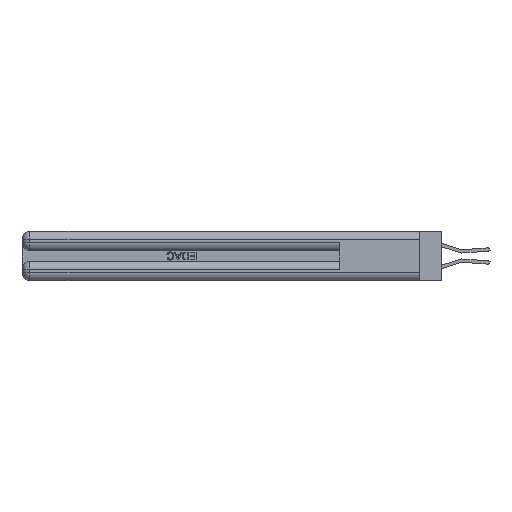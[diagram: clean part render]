
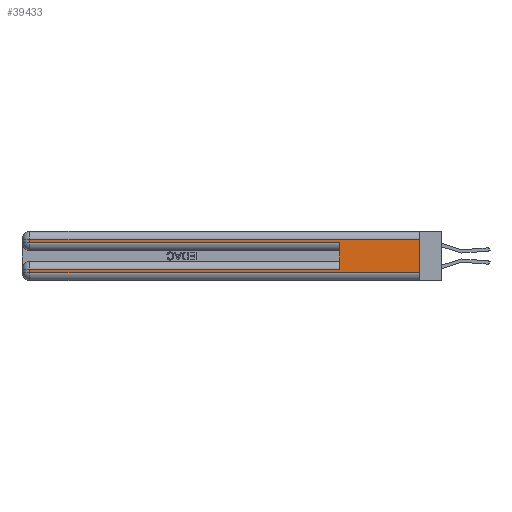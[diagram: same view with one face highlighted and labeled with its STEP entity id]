
A CAD part, left-side view. The second image highlights one B-rep face of the part: STEP entity #39433.
In plain terms, the highlighted planar face has unit normal (-1, 0, 0).
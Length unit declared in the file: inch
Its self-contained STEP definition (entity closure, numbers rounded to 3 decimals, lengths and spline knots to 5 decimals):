
#212 = EDGE_LOOP ( 'NONE', ( #5821, #11777, #9363, #39288, #15627, #4521, #4432, #2448 ) ) ;
#585 = EDGE_CURVE ( 'NONE', #40706, #16194, #4426, .T. ) ;
#684 = VECTOR ( 'NONE', #37307, 39.37008 ) ;
#828 = CARTESIAN_POINT ( 'NONE',  ( 0., 0., 0.06 ) ) ;
#2060 = VERTEX_POINT ( 'NONE', #25319 ) ;
#2448 = ORIENTED_EDGE ( 'NONE', *, *, #4503, .T. ) ;
#3574 = LINE ( 'NONE', #6690, #38582 ) ;
#3845 = CARTESIAN_POINT ( 'NONE',  ( 0., 0.6, 0.145 ) ) ;
#4426 = LINE ( 'NONE', #31833, #6719 ) ;
#4432 = ORIENTED_EDGE ( 'NONE', *, *, #28963, .T. ) ;
#4503 = EDGE_CURVE ( 'NONE', #17765, #16194, #44807, .T. ) ;
#4521 = ORIENTED_EDGE ( 'NONE', *, *, #9127, .T. ) ;
#4641 = LINE ( 'NONE', #33483, #684 ) ;
#4909 = DIRECTION ( 'NONE',  ( 0., -1., 0. ) ) ;
#5194 = CARTESIAN_POINT ( 'NONE',  ( 0., 0.6, 0.085 ) ) ;
#5243 = VERTEX_POINT ( 'NONE', #29019 ) ;
#5821 = ORIENTED_EDGE ( 'NONE', *, *, #585, .F. ) ;
#6690 = CARTESIAN_POINT ( 'NONE',  ( 0., 2.94, 0.37 ) ) ;
#6719 = VECTOR ( 'NONE', #18089, 39.37008 ) ;
#7585 = VECTOR ( 'NONE', #30262, 39.37008 ) ;
#8351 = VERTEX_POINT ( 'NONE', #16807 ) ;
#8817 = CARTESIAN_POINT ( 'NONE',  ( 0., 0., 0.285 ) ) ;
#9003 = VECTOR ( 'NONE', #21394, 39.37008 ) ;
#9127 = EDGE_CURVE ( 'NONE', #21101, #5243, #4641, .T. ) ;
#9363 = ORIENTED_EDGE ( 'NONE', *, *, #11180, .T. ) ;
#11180 = EDGE_CURVE ( 'NONE', #25715, #2060, #43807, .T. ) ;
#11777 = ORIENTED_EDGE ( 'NONE', *, *, #38386, .T. ) ;
#13094 = VECTOR ( 'NONE', #4909, 39.37008 ) ;
#15627 = ORIENTED_EDGE ( 'NONE', *, *, #40161, .F. ) ;
#15644 = VECTOR ( 'NONE', #36802, 39.37008 ) ;
#15941 = VECTOR ( 'NONE', #24783, 39.37008 ) ;
#16194 = VERTEX_POINT ( 'NONE', #828 ) ;
#16807 = CARTESIAN_POINT ( 'NONE',  ( 0., 0.6, 0.285 ) ) ;
#17201 = CARTESIAN_POINT ( 'NONE',  ( 0., 0., 0.06 ) ) ;
#17765 = VERTEX_POINT ( 'NONE', #37957 ) ;
#18089 = DIRECTION ( 'NONE',  ( 0., 0., -1. ) ) ;
#18443 = LINE ( 'NONE', #3845, #15644 ) ;
#21101 = VERTEX_POINT ( 'NONE', #5194 ) ;
#21394 = DIRECTION ( 'NONE',  ( 0., 1., 0. ) ) ;
#22194 = CARTESIAN_POINT ( 'NONE',  ( 0., 2.94, 0.37 ) ) ;
#24700 = DIRECTION ( 'NONE',  ( 0., 0., -1. ) ) ;
#24783 = DIRECTION ( 'NONE',  ( 0., -1., 0. ) ) ;
#24889 = CARTESIAN_POINT ( 'NONE',  ( 0., 0., 0.31 ) ) ;
#25319 = CARTESIAN_POINT ( 'NONE',  ( 0., 2.94, 0.285 ) ) ;
#25715 = VERTEX_POINT ( 'NONE', #43139 ) ;
#28435 = CARTESIAN_POINT ( 'NONE',  ( 0., 0., 0.31 ) ) ;
#28963 = EDGE_CURVE ( 'NONE', #5243, #17765, #3574, .T. ) ;
#29019 = CARTESIAN_POINT ( 'NONE',  ( 0., 2.94, 0.085 ) ) ;
#29326 = EDGE_CURVE ( 'NONE', #2060, #8351, #46536, .T. ) ;
#30262 = DIRECTION ( 'NONE',  ( 0., 0., -1. ) ) ;
#31670 = DIRECTION ( 'NONE',  ( 0., 0., -1. ) ) ;
#31833 = CARTESIAN_POINT ( 'NONE',  ( 0., 0., 0.37 ) ) ;
#32301 = PLANE ( 'NONE',  #34263 ) ;
#32722 = LINE ( 'NONE', #24889, #9003 ) ;
#33483 = CARTESIAN_POINT ( 'NONE',  ( 0., 0., 0.085 ) ) ;
#34263 = AXIS2_PLACEMENT_3D ( 'NONE', #39131, #46766, #31670 ) ;
#34352 = FACE_OUTER_BOUND ( 'NONE', #212, .T. ) ;
#36802 = DIRECTION ( 'NONE',  ( 0., 0., 1. ) ) ;
#37307 = DIRECTION ( 'NONE',  ( 0., 1., 0. ) ) ;
#37957 = CARTESIAN_POINT ( 'NONE',  ( 0., 2.94, 0.06 ) ) ;
#38386 = EDGE_CURVE ( 'NONE', #40706, #25715, #32722, .T. ) ;
#38582 = VECTOR ( 'NONE', #24700, 39.37008 ) ;
#39131 = CARTESIAN_POINT ( 'NONE',  ( 0., 0., 0.37 ) ) ;
#39288 = ORIENTED_EDGE ( 'NONE', *, *, #29326, .T. ) ;
#39433 = ADVANCED_FACE ( 'NONE', ( #34352 ), #32301, .F. ) ;
#40161 = EDGE_CURVE ( 'NONE', #21101, #8351, #18443, .T. ) ;
#40706 = VERTEX_POINT ( 'NONE', #28435 ) ;
#43139 = CARTESIAN_POINT ( 'NONE',  ( 0., 2.94, 0.31 ) ) ;
#43807 = LINE ( 'NONE', #22194, #7585 ) ;
#44807 = LINE ( 'NONE', #17201, #15941 ) ;
#46536 = LINE ( 'NONE', #8817, #13094 ) ;
#46766 = DIRECTION ( 'NONE',  ( 1., 0., 0. ) ) ;
